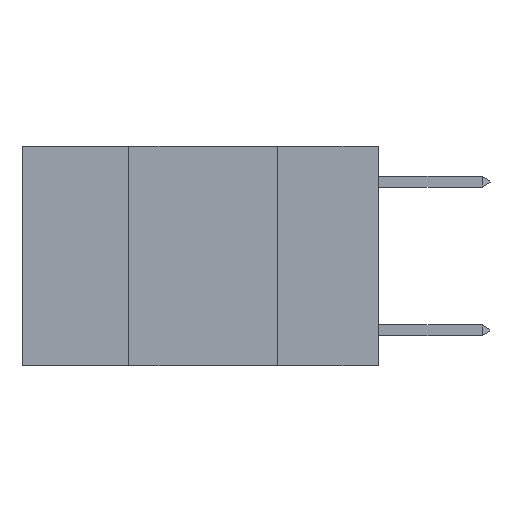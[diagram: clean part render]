
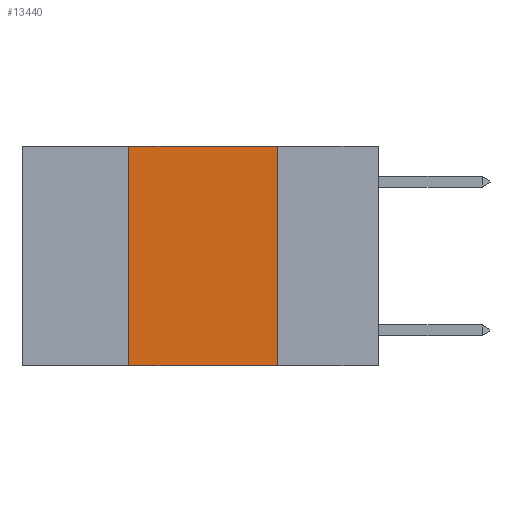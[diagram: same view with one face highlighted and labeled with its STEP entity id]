
A CAD part, left-side view. The second image highlights one B-rep face of the part: STEP entity #13440.
In plain terms, the highlighted planar face has unit normal (-1, 0, 0).
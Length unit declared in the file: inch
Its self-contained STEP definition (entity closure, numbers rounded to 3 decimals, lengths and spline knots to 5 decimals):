
#241 = EDGE_CURVE ( 'NONE', #6884, #3590, #5597, .T. ) ;
#718 = DIRECTION ( 'NONE',  ( 0., -1., 0. ) ) ;
#854 = VECTOR ( 'NONE', #7433, 39.37008 ) ;
#1238 = LINE ( 'NONE', #13272, #10212 ) ;
#1577 = VECTOR ( 'NONE', #7901, 39.37008 ) ;
#1646 = AXIS2_PLACEMENT_3D ( 'NONE', #7793, #4457, #3176 ) ;
#1743 = FACE_OUTER_BOUND ( 'NONE', #2933, .T. ) ;
#2933 = EDGE_LOOP ( 'NONE', ( #14767, #12125, #6482, #7040 ) ) ;
#3176 = DIRECTION ( 'NONE',  ( 0., 0., -1. ) ) ;
#3282 = CARTESIAN_POINT ( 'NONE',  ( 0., 0.6, -0.37 ) ) ;
#3590 = VERTEX_POINT ( 'NONE', #15650 ) ;
#4140 = EDGE_CURVE ( 'NONE', #4188, #10534, #4308, .T. ) ;
#4188 = VERTEX_POINT ( 'NONE', #13937 ) ;
#4301 = PLANE ( 'NONE',  #1646 ) ;
#4308 = LINE ( 'NONE', #5744, #9876 ) ;
#4457 = DIRECTION ( 'NONE',  ( 1., 0., 0. ) ) ;
#5597 = LINE ( 'NONE', #3282, #1577 ) ;
#5744 = CARTESIAN_POINT ( 'NONE',  ( 0., 0.6, 0. ) ) ;
#6342 = EDGE_CURVE ( 'NONE', #10534, #3590, #1238, .T. ) ;
#6402 = LINE ( 'NONE', #14871, #854 ) ;
#6482 = ORIENTED_EDGE ( 'NONE', *, *, #7827, .F. ) ;
#6884 = VERTEX_POINT ( 'NONE', #11922 ) ;
#7040 = ORIENTED_EDGE ( 'NONE', *, *, #241, .T. ) ;
#7433 = DIRECTION ( 'NONE',  ( 0., 0., 1. ) ) ;
#7793 = CARTESIAN_POINT ( 'NONE',  ( 0., 0.6, 0. ) ) ;
#7827 = EDGE_CURVE ( 'NONE', #6884, #4188, #6402, .T. ) ;
#7901 = DIRECTION ( 'NONE',  ( 0., -1., 0. ) ) ;
#9876 = VECTOR ( 'NONE', #718, 39.37008 ) ;
#10212 = VECTOR ( 'NONE', #12099, 39.37008 ) ;
#10534 = VERTEX_POINT ( 'NONE', #11247 ) ;
#11247 = CARTESIAN_POINT ( 'NONE',  ( 0., 0.17, 0. ) ) ;
#11922 = CARTESIAN_POINT ( 'NONE',  ( 0., 0.42, -0.37 ) ) ;
#12099 = DIRECTION ( 'NONE',  ( 0., 0., -1. ) ) ;
#12125 = ORIENTED_EDGE ( 'NONE', *, *, #4140, .F. ) ;
#13272 = CARTESIAN_POINT ( 'NONE',  ( 0., 0.17, 0. ) ) ;
#13440 = ADVANCED_FACE ( 'NONE', ( #1743 ), #4301, .F. ) ;
#13937 = CARTESIAN_POINT ( 'NONE',  ( 0., 0.42, 0. ) ) ;
#14767 = ORIENTED_EDGE ( 'NONE', *, *, #6342, .F. ) ;
#14871 = CARTESIAN_POINT ( 'NONE',  ( 0., 0.42, 0. ) ) ;
#15650 = CARTESIAN_POINT ( 'NONE',  ( 0., 0.17, -0.37 ) ) ;
